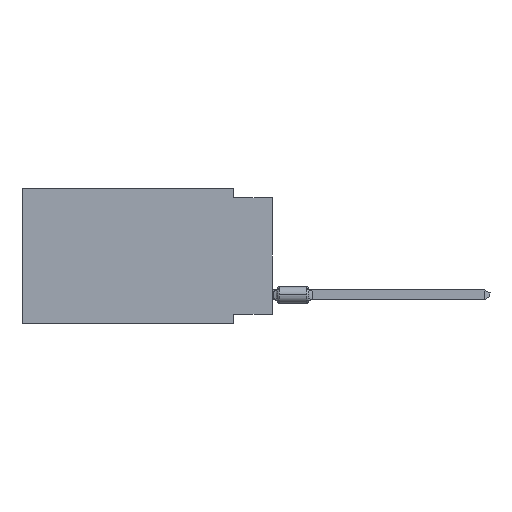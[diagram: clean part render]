
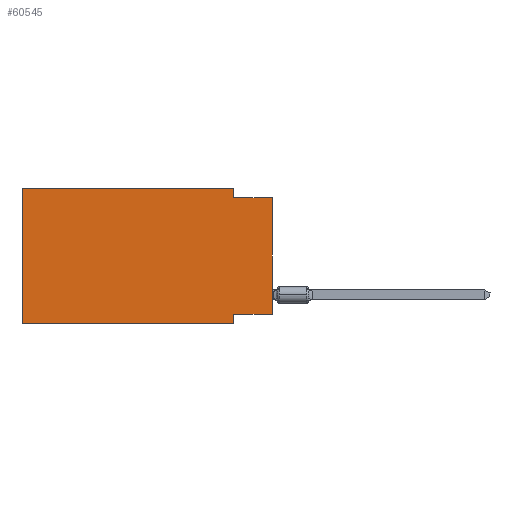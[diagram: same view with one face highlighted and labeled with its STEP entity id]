
A CAD part, left-side view. The second image highlights one B-rep face of the part: STEP entity #60545.
In plain terms, the highlighted planar face has unit normal (-1, 0, 0).
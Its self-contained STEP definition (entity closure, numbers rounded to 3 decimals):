
#267 = VECTOR ( 'NONE', #59054, 1000. ) ;
#915 = LINE ( 'NONE', #15806, #51517 ) ;
#3746 = EDGE_LOOP ( 'NONE', ( #67519, #64943, #91295, #44392, #50188, #68200, #76553, #97045 ) ) ;
#4448 = CARTESIAN_POINT ( 'NONE',  ( 0., 2.54, 0. ) ) ;
#5850 = VERTEX_POINT ( 'NONE', #14251 ) ;
#6403 = DIRECTION ( 'NONE',  ( 0., 0., -1. ) ) ;
#6482 = EDGE_CURVE ( 'NONE', #5850, #54229, #47345, .T. ) ;
#7448 = CARTESIAN_POINT ( 'NONE',  ( 0., 2.54, 0. ) ) ;
#9815 = DIRECTION ( 'NONE',  ( 0., 0., 1. ) ) ;
#9826 = CARTESIAN_POINT ( 'NONE',  ( 0., 16.383, 0. ) ) ;
#11325 = VERTEX_POINT ( 'NONE', #7448 ) ;
#13949 = CARTESIAN_POINT ( 'NONE',  ( 0., 0., -8.255 ) ) ;
#14032 = DIRECTION ( 'NONE',  ( 0., 0., -1. ) ) ;
#14251 = CARTESIAN_POINT ( 'NONE',  ( 0., 2.54, -0.635 ) ) ;
#15806 = CARTESIAN_POINT ( 'NONE',  ( 0., 0., 0. ) ) ;
#16623 = EDGE_CURVE ( 'NONE', #91618, #69652, #89291, .T. ) ;
#17234 = VERTEX_POINT ( 'NONE', #67333 ) ;
#18415 = AXIS2_PLACEMENT_3D ( 'NONE', #91243, #32185, #31694 ) ;
#21858 = EDGE_CURVE ( 'NONE', #69652, #17234, #76511, .T. ) ;
#31212 = PLANE ( 'NONE',  #18415 ) ;
#31694 = DIRECTION ( 'NONE',  ( 0., 0., -1. ) ) ;
#32185 = DIRECTION ( 'NONE',  ( 1., 0., 0. ) ) ;
#32953 = CARTESIAN_POINT ( 'NONE',  ( 0., 0., -0.635 ) ) ;
#36208 = CARTESIAN_POINT ( 'NONE',  ( 0., 0., -8.255 ) ) ;
#40869 = DIRECTION ( 'NONE',  ( 0., -1., 0. ) ) ;
#42590 = EDGE_CURVE ( 'NONE', #11325, #5850, #43646, .T. ) ;
#43646 = LINE ( 'NONE', #4448, #66858 ) ;
#44169 = EDGE_CURVE ( 'NONE', #52118, #17234, #79730, .T. ) ;
#44392 = ORIENTED_EDGE ( 'NONE', *, *, #56628, .F. ) ;
#47345 = LINE ( 'NONE', #32953, #80151 ) ;
#50188 = ORIENTED_EDGE ( 'NONE', *, *, #94363, .F. ) ;
#51517 = VECTOR ( 'NONE', #9815, 1000. ) ;
#52118 = VERTEX_POINT ( 'NONE', #65953 ) ;
#54229 = VERTEX_POINT ( 'NONE', #90475 ) ;
#55898 = CARTESIAN_POINT ( 'NONE',  ( 0., 16.383, 0. ) ) ;
#55930 = CARTESIAN_POINT ( 'NONE',  ( 0., 16.383, -8.89 ) ) ;
#56628 = EDGE_CURVE ( 'NONE', #90038, #11325, #71789, .T. ) ;
#57879 = VECTOR ( 'NONE', #14032, 1000. ) ;
#59054 = DIRECTION ( 'NONE',  ( 0., 1., 0. ) ) ;
#59445 = EDGE_CURVE ( 'NONE', #91618, #54229, #915, .T. ) ;
#60545 = ADVANCED_FACE ( 'NONE', ( #77343 ), #31212, .F. ) ;
#62422 = DIRECTION ( 'NONE',  ( 0., -1., 0. ) ) ;
#62952 = CARTESIAN_POINT ( 'NONE',  ( 0., 2.54, -8.255 ) ) ;
#64329 = LINE ( 'NONE', #55898, #85494 ) ;
#64362 = CARTESIAN_POINT ( 'NONE',  ( 0., 16.383, 0. ) ) ;
#64943 = ORIENTED_EDGE ( 'NONE', *, *, #6482, .F. ) ;
#65953 = CARTESIAN_POINT ( 'NONE',  ( 0., 16.383, -8.89 ) ) ;
#66858 = VECTOR ( 'NONE', #6403, 1000. ) ;
#67333 = CARTESIAN_POINT ( 'NONE',  ( 0., 2.54, -8.89 ) ) ;
#67519 = ORIENTED_EDGE ( 'NONE', *, *, #59445, .T. ) ;
#68200 = ORIENTED_EDGE ( 'NONE', *, *, #44169, .T. ) ;
#69652 = VERTEX_POINT ( 'NONE', #62952 ) ;
#71789 = LINE ( 'NONE', #64362, #78030 ) ;
#76511 = LINE ( 'NONE', #97869, #57879 ) ;
#76553 = ORIENTED_EDGE ( 'NONE', *, *, #21858, .F. ) ;
#77343 = FACE_OUTER_BOUND ( 'NONE', #3746, .T. ) ;
#78030 = VECTOR ( 'NONE', #62422, 1000. ) ;
#79730 = LINE ( 'NONE', #55930, #89538 ) ;
#80151 = VECTOR ( 'NONE', #40869, 1000. ) ;
#85494 = VECTOR ( 'NONE', #86163, 1000. ) ;
#86163 = DIRECTION ( 'NONE',  ( 0., 0., 1. ) ) ;
#89291 = LINE ( 'NONE', #36208, #267 ) ;
#89538 = VECTOR ( 'NONE', #95585, 1000. ) ;
#90038 = VERTEX_POINT ( 'NONE', #9826 ) ;
#90475 = CARTESIAN_POINT ( 'NONE',  ( 0., 0., -0.635 ) ) ;
#91243 = CARTESIAN_POINT ( 'NONE',  ( 0., 16.383, 0. ) ) ;
#91295 = ORIENTED_EDGE ( 'NONE', *, *, #42590, .F. ) ;
#91618 = VERTEX_POINT ( 'NONE', #13949 ) ;
#94363 = EDGE_CURVE ( 'NONE', #52118, #90038, #64329, .T. ) ;
#95585 = DIRECTION ( 'NONE',  ( 0., -1., 0. ) ) ;
#97045 = ORIENTED_EDGE ( 'NONE', *, *, #16623, .F. ) ;
#97869 = CARTESIAN_POINT ( 'NONE',  ( 0., 2.54, -8.89 ) ) ;
